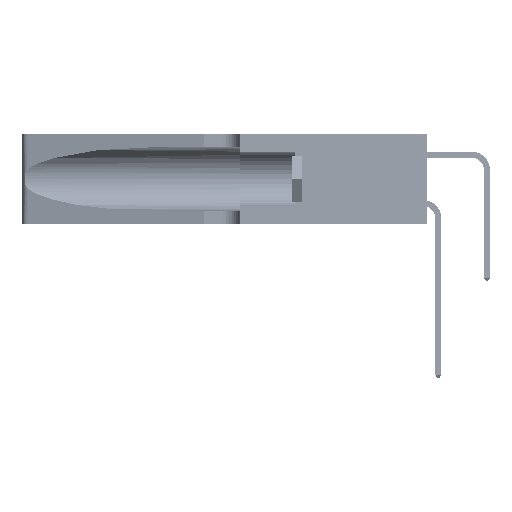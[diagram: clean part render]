
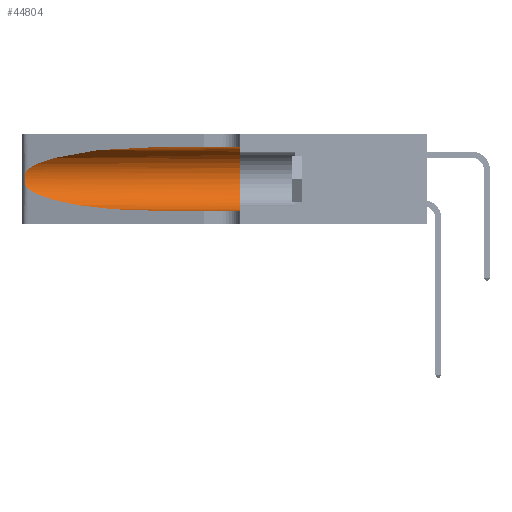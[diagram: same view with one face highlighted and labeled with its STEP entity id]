
A CAD part, left-side view. The second image highlights one B-rep face of the part: STEP entity #44804.
In plain terms, the highlighted cylindrical face has radius 3.308 mm (diameter 6.617 mm), a partial arc.
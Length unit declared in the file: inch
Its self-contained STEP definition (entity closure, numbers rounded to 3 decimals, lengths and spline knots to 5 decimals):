
#317 = CARTESIAN_POINT ( 'NONE',  ( 0.25639, 1.23186, 0.15144 ) ) ;
#323 = B_SPLINE_CURVE_WITH_KNOTS ( 'NONE', 3,
 ( #40744, #4346, #8472, #36898, #12614, #40913, #16743, #44953, #20823, #48952, #24908, #317, #28972, #4524 ),
 .UNSPECIFIED., .F., .F.,
 ( 4, 2, 2, 2, 2, 2, 4 ),
 ( 0., 0.00027, 0.00053, 0.00107, 0.0016, 0.00187, 0.00214 ),
 .UNSPECIFIED. ) ;
#652 = ORIENTED_EDGE ( 'NONE', *, *, #19191, .F. ) ;
#1933 = VERTEX_POINT ( 'NONE', #48668 ) ;
#2434 = CARTESIAN_POINT ( 'NONE',  ( 0.1305, 0.35, 0.31525 ) ) ;
#3912 = ORIENTED_EDGE ( 'NONE', *, *, #13065, .T. ) ;
#4346 = CARTESIAN_POINT ( 'NONE',  ( 0.25555, 1.22994, 0.2215 ) ) ;
#4524 = CARTESIAN_POINT ( 'NONE',  ( 0.25487, 1.22718, 0.14631 ) ) ;
#4755 = LINE ( 'NONE', #34673, #37215 ) ;
#7396 = CARTESIAN_POINT ( 'NONE',  ( 0.2373, 1.15595, 0.08982 ) ) ;
#8472 = CARTESIAN_POINT ( 'NONE',  ( 0.25639, 1.23184, 0.21858 ) ) ;
#8483 = CARTESIAN_POINT ( 'NONE',  ( 0.18966, 0.96281, 0.31525 ) ) ;
#9332 = VECTOR ( 'NONE', #24857, 39.37008 ) ;
#9660 = ORIENTED_EDGE ( 'NONE', *, *, #39195, .T. ) ;
#9942 =( BOUNDED_CURVE ( )  B_SPLINE_CURVE ( 3, ( #32858, #8483, #44963, #20833 ),
 .UNSPECIFIED., .F., .F. ) 
 B_SPLINE_CURVE_WITH_KNOTS ( ( 4, 4 ),
 ( 1.5708, 2.84003 ),
 .UNSPECIFIED. ) 
 CURVE ( )  GEOMETRIC_REPRESENTATION_ITEM ( )  RATIONAL_B_SPLINE_CURVE ( ( 1., 0.87, 0.87, 1. ) ) 
 REPRESENTATION_ITEM ( '' )  );
#10318 = DIRECTION ( 'NONE',  ( 0., -1., 0. ) ) ;
#11087 = CIRCLE ( 'NONE', #31503, 0.13025 ) ;
#11529 = CARTESIAN_POINT ( 'NONE',  ( 0.18966, 0.96281, 0.05475 ) ) ;
#12614 = CARTESIAN_POINT ( 'NONE',  ( 0.25854, 1.2359, 0.20912 ) ) ;
#13065 = EDGE_CURVE ( 'NONE', #39826, #18867, #42104, .T. ) ;
#14467 = FACE_OUTER_BOUND ( 'NONE', #21175, .T. ) ;
#15791 = LINE ( 'NONE', #28763, #9332 ) ;
#16743 = CARTESIAN_POINT ( 'NONE',  ( 0.26075, 1.23896, 0.19203 ) ) ;
#18867 = VERTEX_POINT ( 'NONE', #24660 ) ;
#19191 = EDGE_CURVE ( 'NONE', #49075, #38524, #4755, .T. ) ;
#20520 = DIRECTION ( 'NONE',  ( 0., 1., 0. ) ) ;
#20823 = CARTESIAN_POINT ( 'NONE',  ( 0.26017, 1.23833, 0.17102 ) ) ;
#20833 = CARTESIAN_POINT ( 'NONE',  ( 0.25487, 1.22718, 0.22369 ) ) ;
#21175 = EDGE_LOOP ( 'NONE', ( #9660, #35131, #3912, #38875, #29452, #652 ) ) ;
#23022 = DIRECTION ( 'NONE',  ( 0., 0., -1. ) ) ;
#23638 = EDGE_CURVE ( 'NONE', #18867, #44004, #15791, .T. ) ;
#24063 = CYLINDRICAL_SURFACE ( 'NONE', #34839, 0.13025 ) ;
#24660 = CARTESIAN_POINT ( 'NONE',  ( 0.1305, 0.72297, 0.05475 ) ) ;
#24857 = DIRECTION ( 'NONE',  ( 0., -1., 0. ) ) ;
#24908 = CARTESIAN_POINT ( 'NONE',  ( 0.25789, 1.23486, 0.15765 ) ) ;
#27088 = DIRECTION ( 'NONE',  ( 0., -1., 0. ) ) ;
#28763 = CARTESIAN_POINT ( 'NONE',  ( 0.1305, 1.61858, 0.05475 ) ) ;
#28972 = CARTESIAN_POINT ( 'NONE',  ( 0.25555, 1.22993, 0.14849 ) ) ;
#29452 = ORIENTED_EDGE ( 'NONE', *, *, #35625, .F. ) ;
#31503 = AXIS2_PLACEMENT_3D ( 'NONE', #44656, #20520, #48659 ) ;
#32858 = CARTESIAN_POINT ( 'NONE',  ( 0.1305, 0.72297, 0.31525 ) ) ;
#34673 = CARTESIAN_POINT ( 'NONE',  ( 0.1305, 1.61858, 0.31525 ) ) ;
#34839 = AXIS2_PLACEMENT_3D ( 'NONE', #51094, #27088, #23022 ) ;
#35131 = ORIENTED_EDGE ( 'NONE', *, *, #43214, .T. ) ;
#35625 = EDGE_CURVE ( 'NONE', #38524, #44004, #11087, .T. ) ;
#35821 = CARTESIAN_POINT ( 'NONE',  ( 0.1305, 0.72297, 0.31525 ) ) ;
#36898 = CARTESIAN_POINT ( 'NONE',  ( 0.25787, 1.23484, 0.2124 ) ) ;
#37215 = VECTOR ( 'NONE', #10318, 39.37008 ) ;
#38524 = VERTEX_POINT ( 'NONE', #2434 ) ;
#38875 = ORIENTED_EDGE ( 'NONE', *, *, #23638, .T. ) ;
#39195 = EDGE_CURVE ( 'NONE', #49075, #1933, #9942, .T. ) ;
#39826 = VERTEX_POINT ( 'NONE', #40856 ) ;
#39850 = CARTESIAN_POINT ( 'NONE',  ( 0.25487, 1.22718, 0.14631 ) ) ;
#40744 = CARTESIAN_POINT ( 'NONE',  ( 0.25487, 1.22718, 0.22369 ) ) ;
#40856 = CARTESIAN_POINT ( 'NONE',  ( 0.25487, 1.22718, 0.14631 ) ) ;
#40913 = CARTESIAN_POINT ( 'NONE',  ( 0.26018, 1.23835, 0.19895 ) ) ;
#41533 = CARTESIAN_POINT ( 'NONE',  ( 0.1305, 0.35, 0.05475 ) ) ;
#42104 =( BOUNDED_CURVE ( )  B_SPLINE_CURVE ( 3, ( #39850, #7396, #11529, #43911 ),
 .UNSPECIFIED., .F., .F. ) 
 B_SPLINE_CURVE_WITH_KNOTS ( ( 4, 4 ),
 ( 3.44316, 4.71239 ),
 .UNSPECIFIED. ) 
 CURVE ( )  GEOMETRIC_REPRESENTATION_ITEM ( )  RATIONAL_B_SPLINE_CURVE ( ( 1., 0.87, 0.87, 1. ) ) 
 REPRESENTATION_ITEM ( '' )  );
#43214 = EDGE_CURVE ( 'NONE', #1933, #39826, #323, .T. ) ;
#43911 = CARTESIAN_POINT ( 'NONE',  ( 0.1305, 0.72297, 0.05475 ) ) ;
#44004 = VERTEX_POINT ( 'NONE', #41533 ) ;
#44656 = CARTESIAN_POINT ( 'NONE',  ( 0.1305, 0.35, 0.185 ) ) ;
#44804 = ADVANCED_FACE ( 'NONE', ( #14467 ), #24063, .F. ) ;
#44953 = CARTESIAN_POINT ( 'NONE',  ( 0.26075, 1.23896, 0.178 ) ) ;
#44963 = CARTESIAN_POINT ( 'NONE',  ( 0.2373, 1.15595, 0.28018 ) ) ;
#48659 = DIRECTION ( 'NONE',  ( 0., 0., 1. ) ) ;
#48668 = CARTESIAN_POINT ( 'NONE',  ( 0.25487, 1.22718, 0.22369 ) ) ;
#48952 = CARTESIAN_POINT ( 'NONE',  ( 0.25856, 1.23593, 0.16098 ) ) ;
#49075 = VERTEX_POINT ( 'NONE', #35821 ) ;
#51094 = CARTESIAN_POINT ( 'NONE',  ( 0.1305, 1.61858, 0.185 ) ) ;
